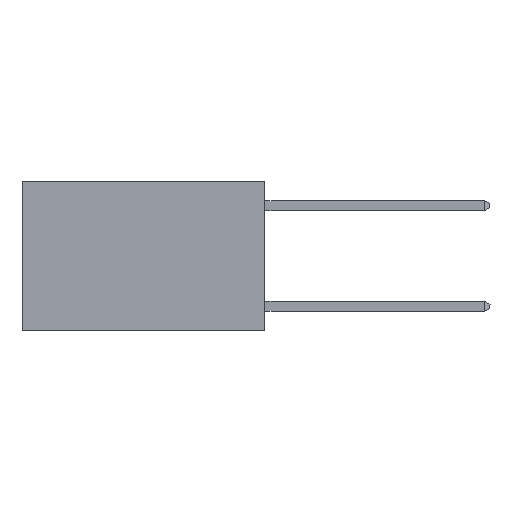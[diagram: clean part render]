
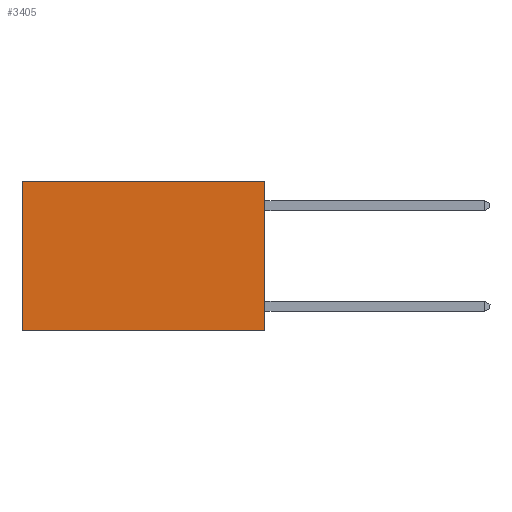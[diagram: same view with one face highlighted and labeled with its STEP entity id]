
A CAD part, left-side view. The second image highlights one B-rep face of the part: STEP entity #3405.
In plain terms, the highlighted planar face has unit normal (-1, 0, 0).
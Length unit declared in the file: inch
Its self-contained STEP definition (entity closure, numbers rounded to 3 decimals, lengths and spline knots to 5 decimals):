
#148 = FACE_OUTER_BOUND ( 'NONE', #427, .T. ) ;
#177 = DIRECTION ( 'NONE',  ( 0., 0., -1. ) ) ;
#266 = DIRECTION ( 'NONE',  ( 1., 0., 0. ) ) ;
#330 = CARTESIAN_POINT ( 'NONE',  ( 0.2625, 0., -0.37 ) ) ;
#427 = EDGE_LOOP ( 'NONE', ( #2456, #4878, #6889, #5336 ) ) ;
#546 = VECTOR ( 'NONE', #1416, 39.37008 ) ;
#848 = VERTEX_POINT ( 'NONE', #1285 ) ;
#1053 = CARTESIAN_POINT ( 'NONE',  ( 0.2625, 0., 0. ) ) ;
#1285 = CARTESIAN_POINT ( 'NONE',  ( 0.2625, 0., 0. ) ) ;
#1416 = DIRECTION ( 'NONE',  ( 0., 1., 0. ) ) ;
#1551 = LINE ( 'NONE', #5940, #9400 ) ;
#1776 = VERTEX_POINT ( 'NONE', #9002 ) ;
#2224 = LINE ( 'NONE', #4886, #8347 ) ;
#2456 = ORIENTED_EDGE ( 'NONE', *, *, #3811, .T. ) ;
#2701 = AXIS2_PLACEMENT_3D ( 'NONE', #1053, #266, #6013 ) ;
#3146 = VECTOR ( 'NONE', #3799, 39.37008 ) ;
#3175 = CARTESIAN_POINT ( 'NONE',  ( 0.2625, 0., 0. ) ) ;
#3251 = EDGE_CURVE ( 'NONE', #848, #4801, #8565, .T. ) ;
#3297 = EDGE_CURVE ( 'NONE', #848, #1776, #2224, .T. ) ;
#3405 = ADVANCED_FACE ( 'NONE', ( #148 ), #9460, .F. ) ;
#3799 = DIRECTION ( 'NONE',  ( 0., 1., 0. ) ) ;
#3811 = EDGE_CURVE ( 'NONE', #4801, #4604, #1551, .T. ) ;
#4604 = VERTEX_POINT ( 'NONE', #7501 ) ;
#4801 = VERTEX_POINT ( 'NONE', #6329 ) ;
#4878 = ORIENTED_EDGE ( 'NONE', *, *, #6575, .F. ) ;
#4886 = CARTESIAN_POINT ( 'NONE',  ( 0.2625, 0., 0. ) ) ;
#5336 = ORIENTED_EDGE ( 'NONE', *, *, #3251, .T. ) ;
#5940 = CARTESIAN_POINT ( 'NONE',  ( 0.2625, 0.6, 0. ) ) ;
#6013 = DIRECTION ( 'NONE',  ( 0., 0., -1. ) ) ;
#6329 = CARTESIAN_POINT ( 'NONE',  ( 0.2625, 0.6, 0. ) ) ;
#6575 = EDGE_CURVE ( 'NONE', #1776, #4604, #7200, .T. ) ;
#6889 = ORIENTED_EDGE ( 'NONE', *, *, #3297, .F. ) ;
#7200 = LINE ( 'NONE', #330, #3146 ) ;
#7501 = CARTESIAN_POINT ( 'NONE',  ( 0.2625, 0.6, -0.37 ) ) ;
#8347 = VECTOR ( 'NONE', #8422, 39.37008 ) ;
#8422 = DIRECTION ( 'NONE',  ( 0., 0., -1. ) ) ;
#8565 = LINE ( 'NONE', #3175, #546 ) ;
#9002 = CARTESIAN_POINT ( 'NONE',  ( 0.2625, 0., -0.37 ) ) ;
#9400 = VECTOR ( 'NONE', #177, 39.37008 ) ;
#9460 = PLANE ( 'NONE',  #2701 ) ;
